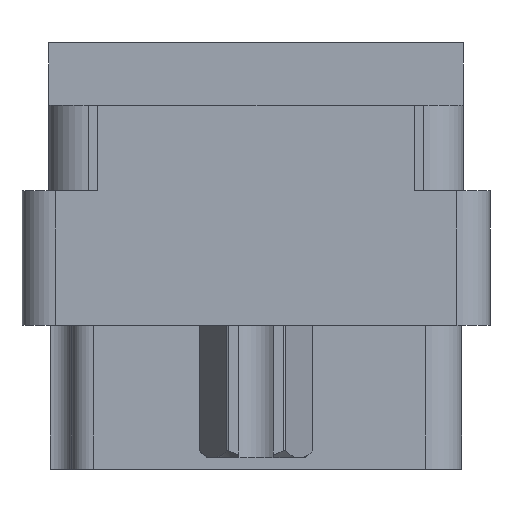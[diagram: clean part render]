
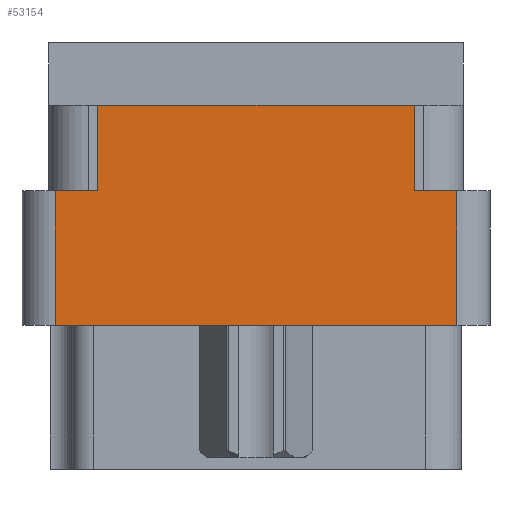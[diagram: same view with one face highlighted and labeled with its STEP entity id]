
A CAD part, left-side view. The second image highlights one B-rep face of the part: STEP entity #53154.
In plain terms, the highlighted planar face has unit normal (-1, 0, 0).
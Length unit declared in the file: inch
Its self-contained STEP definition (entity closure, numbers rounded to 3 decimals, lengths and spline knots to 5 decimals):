
#221 = EDGE_CURVE ( 'NONE', #33065, #11679, #3452, .T. ) ;
#463 = DIRECTION ( 'NONE',  ( 0., 0., 1. ) ) ;
#1826 = ORIENTED_EDGE ( 'NONE', *, *, #18301, .F. ) ;
#3452 = LINE ( 'NONE', #15269, #12159 ) ;
#4731 = CARTESIAN_POINT ( 'NONE',  ( -1.296, 0.296, -0.277 ) ) ;
#4880 = EDGE_CURVE ( 'NONE', #36366, #49020, #4977, .T. ) ;
#4977 = LINE ( 'NONE', #52777, #49136 ) ;
#5519 = ORIENTED_EDGE ( 'NONE', *, *, #4880, .T. ) ;
#6357 = CARTESIAN_POINT ( 'NONE',  ( -1.296, 0.296, -0.277 ) ) ;
#7796 = DIRECTION ( 'NONE',  ( 0., -1., 0. ) ) ;
#8464 = VERTEX_POINT ( 'NONE', #41234 ) ;
#8786 = AXIS2_PLACEMENT_3D ( 'NONE', #12670, #29895, #463 ) ;
#9002 = VECTOR ( 'NONE', #7796, 39.37008 ) ;
#9788 = CARTESIAN_POINT ( 'NONE',  ( -1.296, 0., -0.529 ) ) ;
#10985 = LINE ( 'NONE', #50425, #9002 ) ;
#11361 = LINE ( 'NONE', #43551, #33500 ) ;
#11545 = ORIENTED_EDGE ( 'NONE', *, *, #21489, .F. ) ;
#11679 = VERTEX_POINT ( 'NONE', #53802 ) ;
#12159 = VECTOR ( 'NONE', #53933, 39.37008 ) ;
#12670 = CARTESIAN_POINT ( 'NONE',  ( -1.296, -0.438, -0.798 ) ) ;
#13749 = DIRECTION ( 'NONE',  ( 0., -1., 0. ) ) ;
#15135 = DIRECTION ( 'NONE',  ( 0., 0., 1. ) ) ;
#15269 = CARTESIAN_POINT ( 'NONE',  ( -1.296, 0.376, -0.798 ) ) ;
#15342 = CARTESIAN_POINT ( 'NONE',  ( -1.296, -0.376, -0.277 ) ) ;
#16962 = VECTOR ( 'NONE', #29555, 39.37008 ) ;
#17140 = PLANE ( 'NONE',  #8786 ) ;
#17539 = LINE ( 'NONE', #49874, #27583 ) ;
#18301 = EDGE_CURVE ( 'NONE', #33065, #28507, #11361, .T. ) ;
#21489 = EDGE_CURVE ( 'NONE', #30266, #11679, #49087, .T. ) ;
#21920 = DIRECTION ( 'NONE',  ( 0., 0., 1. ) ) ;
#22001 = ORIENTED_EDGE ( 'NONE', *, *, #31280, .F. ) ;
#22366 = CARTESIAN_POINT ( 'NONE',  ( -1.296, -0.296, -0.117 ) ) ;
#22370 = CARTESIAN_POINT ( 'NONE',  ( -1.296, 0.376, -0.277 ) ) ;
#22766 = EDGE_CURVE ( 'NONE', #30266, #25472, #17539, .T. ) ;
#23621 = LINE ( 'NONE', #4731, #29015 ) ;
#25472 = VERTEX_POINT ( 'NONE', #15342 ) ;
#26085 = ORIENTED_EDGE ( 'NONE', *, *, #221, .T. ) ;
#26495 = CARTESIAN_POINT ( 'NONE',  ( -1.296, -0.376, -0.529 ) ) ;
#27583 = VECTOR ( 'NONE', #15135, 39.37008 ) ;
#28507 = VERTEX_POINT ( 'NONE', #6357 ) ;
#29015 = VECTOR ( 'NONE', #21920, 39.37008 ) ;
#29097 = FACE_OUTER_BOUND ( 'NONE', #36800, .T. ) ;
#29555 = DIRECTION ( 'NONE',  ( 0., -1., 0. ) ) ;
#29895 = DIRECTION ( 'NONE',  ( -1., 0., 0. ) ) ;
#29912 = CARTESIAN_POINT ( 'NONE',  ( -1.296, 0., -0.277 ) ) ;
#30266 = VERTEX_POINT ( 'NONE', #26495 ) ;
#30338 = ORIENTED_EDGE ( 'NONE', *, *, #41164, .F. ) ;
#31280 = EDGE_CURVE ( 'NONE', #28507, #8464, #23621, .T. ) ;
#33040 = LINE ( 'NONE', #29912, #16962 ) ;
#33065 = VERTEX_POINT ( 'NONE', #22370 ) ;
#33500 = VECTOR ( 'NONE', #13749, 39.37008 ) ;
#33725 = ORIENTED_EDGE ( 'NONE', *, *, #53057, .F. ) ;
#35830 = DIRECTION ( 'NONE',  ( 0., 0., 1. ) ) ;
#36366 = VERTEX_POINT ( 'NONE', #52096 ) ;
#36800 = EDGE_LOOP ( 'NONE', ( #1826, #26085, #11545, #52379, #30338, #5519, #33725, #22001 ) ) ;
#37775 = VECTOR ( 'NONE', #39997, 39.37008 ) ;
#39997 = DIRECTION ( 'NONE',  ( 0., 1., 0. ) ) ;
#41164 = EDGE_CURVE ( 'NONE', #36366, #25472, #33040, .T. ) ;
#41234 = CARTESIAN_POINT ( 'NONE',  ( -1.296, 0.296, -0.117 ) ) ;
#43551 = CARTESIAN_POINT ( 'NONE',  ( -1.296, 0., -0.277 ) ) ;
#49020 = VERTEX_POINT ( 'NONE', #22366 ) ;
#49087 = LINE ( 'NONE', #9788, #37775 ) ;
#49136 = VECTOR ( 'NONE', #35830, 39.37008 ) ;
#49874 = CARTESIAN_POINT ( 'NONE',  ( -1.296, -0.376, -0.798 ) ) ;
#50425 = CARTESIAN_POINT ( 'NONE',  ( -1.296, 0.438, -0.117 ) ) ;
#52096 = CARTESIAN_POINT ( 'NONE',  ( -1.296, -0.296, -0.277 ) ) ;
#52379 = ORIENTED_EDGE ( 'NONE', *, *, #22766, .T. ) ;
#52777 = CARTESIAN_POINT ( 'NONE',  ( -1.296, -0.296, -0.277 ) ) ;
#53057 = EDGE_CURVE ( 'NONE', #8464, #49020, #10985, .T. ) ;
#53154 = ADVANCED_FACE ( 'NONE', ( #29097 ), #17140, .T. ) ;
#53802 = CARTESIAN_POINT ( 'NONE',  ( -1.296, 0.376, -0.529 ) ) ;
#53933 = DIRECTION ( 'NONE',  ( 0., 0., -1. ) ) ;
